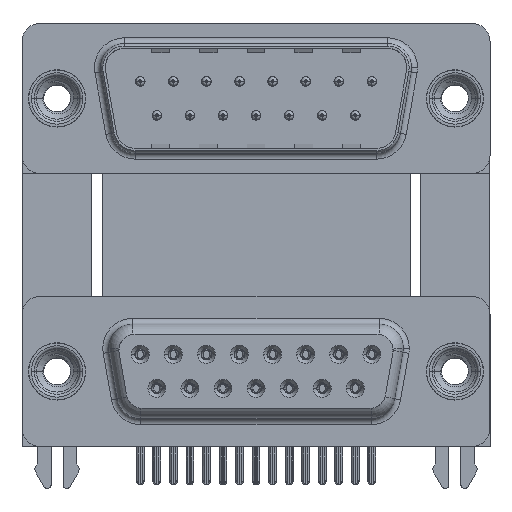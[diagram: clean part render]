
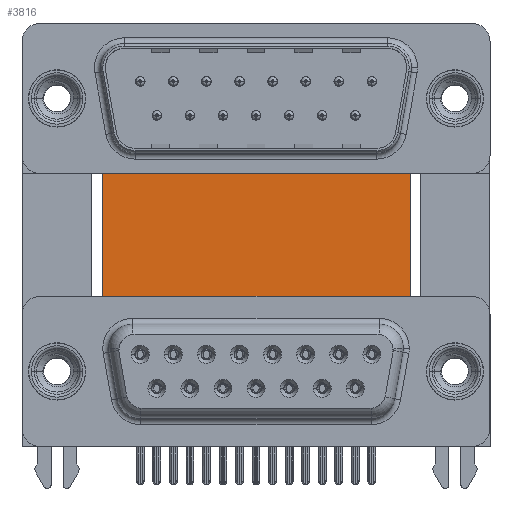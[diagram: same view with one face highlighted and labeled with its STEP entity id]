
A CAD part, top view. The second image highlights one B-rep face of the part: STEP entity #3816.
In plain terms, the highlighted planar face has unit normal (0, 0, 1).
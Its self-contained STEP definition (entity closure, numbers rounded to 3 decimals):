
#1846 = CARTESIAN_POINT ( 'NONE',  ( 3.79, 16.585, -12. ) ) ;
#2273 = EDGE_CURVE ( 'NONE', #9493, #21456, #31810, .T. ) ;
#3809 = ORIENTED_EDGE ( 'NONE', *, *, #2273, .F. ) ;
#3816 = ADVANCED_FACE ( 'NONE', ( #28581 ), #14143, .F. ) ;
#6323 = EDGE_LOOP ( 'NONE', ( #21857, #21013, #3809, #31799 ) ) ;
#7465 = CARTESIAN_POINT ( 'NONE',  ( 29.58, 16.585, -12. ) ) ;
#8434 = LINE ( 'NONE', #36764, #10555 ) ;
#9493 = VERTEX_POINT ( 'NONE', #1846 ) ;
#9609 = CARTESIAN_POINT ( 'NONE',  ( 29.58, -3.735, -12. ) ) ;
#10415 = DIRECTION ( 'NONE',  ( 1., 0., 0. ) ) ;
#10555 = VECTOR ( 'NONE', #33303, 1000. ) ;
#12004 = VECTOR ( 'NONE', #38900, 1000. ) ;
#14143 = PLANE ( 'NONE',  #22836 ) ;
#17177 = CARTESIAN_POINT ( 'NONE',  ( 3.79, 16.585, -12. ) ) ;
#17572 = CARTESIAN_POINT ( 'NONE',  ( 3.79, 16.585, -12. ) ) ;
#21013 = ORIENTED_EDGE ( 'NONE', *, *, #31848, .F. ) ;
#21456 = VERTEX_POINT ( 'NONE', #34430 ) ;
#21600 = DIRECTION ( 'NONE',  ( 0., 0., -1. ) ) ;
#21857 = ORIENTED_EDGE ( 'NONE', *, *, #26955, .T. ) ;
#22836 = AXIS2_PLACEMENT_3D ( 'NONE', #17177, #21600, #24644 ) ;
#23909 = EDGE_CURVE ( 'NONE', #9493, #30086, #42137, .T. ) ;
#24644 = DIRECTION ( 'NONE',  ( -1., 0., 0. ) ) ;
#26955 = EDGE_CURVE ( 'NONE', #30086, #31153, #8434, .T. ) ;
#28581 = FACE_OUTER_BOUND ( 'NONE', #6323, .T. ) ;
#30037 = VECTOR ( 'NONE', #32554, 1000. ) ;
#30086 = VERTEX_POINT ( 'NONE', #33964 ) ;
#31153 = VERTEX_POINT ( 'NONE', #9609 ) ;
#31799 = ORIENTED_EDGE ( 'NONE', *, *, #23909, .T. ) ;
#31810 = LINE ( 'NONE', #45711, #35702 ) ;
#31848 = EDGE_CURVE ( 'NONE', #21456, #31153, #36019, .T. ) ;
#32554 = DIRECTION ( 'NONE',  ( 0., -1., 0. ) ) ;
#33303 = DIRECTION ( 'NONE',  ( 1., 0., 0. ) ) ;
#33964 = CARTESIAN_POINT ( 'NONE',  ( 3.79, -3.735, -12. ) ) ;
#34430 = CARTESIAN_POINT ( 'NONE',  ( 29.58, 16.585, -12. ) ) ;
#35702 = VECTOR ( 'NONE', #10415, 1000. ) ;
#36019 = LINE ( 'NONE', #7465, #30037 ) ;
#36764 = CARTESIAN_POINT ( 'NONE',  ( 3.79, -3.735, -12. ) ) ;
#38900 = DIRECTION ( 'NONE',  ( 0., -1., 0. ) ) ;
#42137 = LINE ( 'NONE', #17572, #12004 ) ;
#45711 = CARTESIAN_POINT ( 'NONE',  ( 3.79, 16.585, -12. ) ) ;
